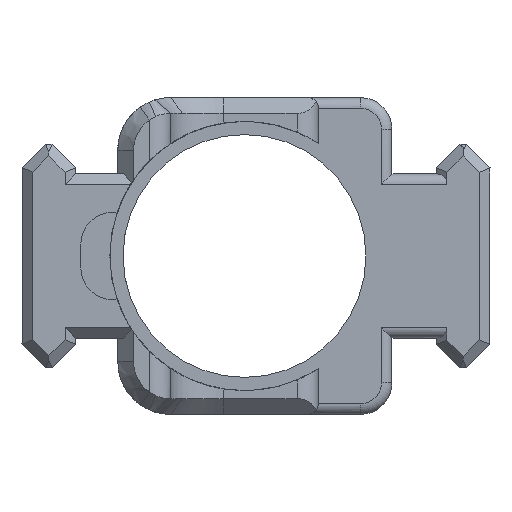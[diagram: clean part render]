
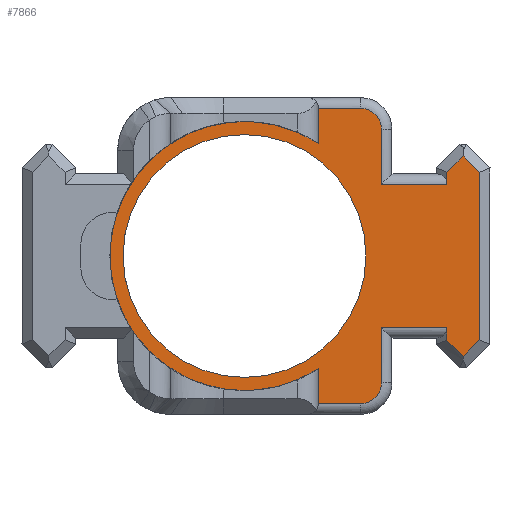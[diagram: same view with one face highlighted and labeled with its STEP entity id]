
A CAD part, left-side view. The second image highlights one B-rep face of the part: STEP entity #7866.
In plain terms, the highlighted planar face has unit normal (-1, 0, 0).
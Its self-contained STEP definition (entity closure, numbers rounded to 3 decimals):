
#35=FACE_BOUND('',#786,.T.);
#176=CIRCLE('',#8368,12.75);
#184=CIRCLE('',#8390,2.);
#185=CIRCLE('',#8391,2.);
#186=CIRCLE('',#8392,11.5);
#327=FACE_OUTER_BOUND('',#785,.T.);
#785=EDGE_LOOP('',(#5769,#5770,#5771,#5772,#5773,#5774,#5775,#5776,#5777,
#5778,#5779,#5780,#5781,#5782,#5783,#5784,#5785,#5786));
#786=EDGE_LOOP('',(#5787));
#1500=LINE('',#12039,#2532);
#1501=LINE('',#12043,#2533);
#1504=LINE('',#12059,#2536);
#1508=LINE('',#12072,#2540);
#1509=LINE('',#12074,#2541);
#1510=LINE('',#12076,#2542);
#1511=LINE('',#12078,#2543);
#1512=LINE('',#12080,#2544);
#1513=LINE('',#12082,#2545);
#1514=LINE('',#12084,#2546);
#1515=LINE('',#12086,#2547);
#1516=LINE('',#12088,#2548);
#1517=LINE('',#12090,#2549);
#1518=LINE('',#12092,#2550);
#1519=LINE('',#12095,#2551);
#2532=VECTOR('',#9451,10.);
#2533=VECTOR('',#9456,10.);
#2536=VECTOR('',#9467,10.);
#2540=VECTOR('',#9481,10.);
#2541=VECTOR('',#9482,10.);
#2542=VECTOR('',#9483,10.);
#2543=VECTOR('',#9484,10.);
#2544=VECTOR('',#9485,10.);
#2545=VECTOR('',#9486,10.);
#2546=VECTOR('',#9487,10.);
#2547=VECTOR('',#9488,10.);
#2548=VECTOR('',#9489,10.);
#2549=VECTOR('',#9490,10.);
#2550=VECTOR('',#9491,10.);
#2551=VECTOR('',#9494,10.);
#3503=VERTEX_POINT('',#11846);
#3510=VERTEX_POINT('',#11880);
#3511=VERTEX_POINT('',#11882);
#3533=VERTEX_POINT('',#12041);
#3536=VERTEX_POINT('',#12053);
#3539=VERTEX_POINT('',#12069);
#3540=VERTEX_POINT('',#12071);
#3541=VERTEX_POINT('',#12073);
#3542=VERTEX_POINT('',#12075);
#3543=VERTEX_POINT('',#12077);
#3544=VERTEX_POINT('',#12079);
#3545=VERTEX_POINT('',#12081);
#3546=VERTEX_POINT('',#12083);
#3547=VERTEX_POINT('',#12085);
#3548=VERTEX_POINT('',#12087);
#3549=VERTEX_POINT('',#12089);
#3550=VERTEX_POINT('',#12091);
#3551=VERTEX_POINT('',#12093);
#3552=VERTEX_POINT('',#12096);
#4323=EDGE_CURVE('',#3510,#3511,#176,.T.);
#4346=EDGE_CURVE('',#3510,#3503,#1500,.T.);
#4348=EDGE_CURVE('',#3533,#3503,#1501,.T.);
#4354=EDGE_CURVE('',#3536,#3511,#1504,.T.);
#4359=EDGE_CURVE('',#3539,#3533,#184,.T.);
#4360=EDGE_CURVE('',#3540,#3539,#1508,.T.);
#4361=EDGE_CURVE('',#3541,#3540,#1509,.T.);
#4362=EDGE_CURVE('',#3542,#3541,#1510,.T.);
#4363=EDGE_CURVE('',#3543,#3542,#1511,.T.);
#4364=EDGE_CURVE('',#3544,#3543,#1512,.T.);
#4365=EDGE_CURVE('',#3545,#3544,#1513,.T.);
#4366=EDGE_CURVE('',#3546,#3545,#1514,.T.);
#4367=EDGE_CURVE('',#3547,#3546,#1515,.T.);
#4368=EDGE_CURVE('',#3548,#3547,#1516,.T.);
#4369=EDGE_CURVE('',#3549,#3548,#1517,.T.);
#4370=EDGE_CURVE('',#3550,#3549,#1518,.T.);
#4371=EDGE_CURVE('',#3551,#3550,#185,.T.);
#4372=EDGE_CURVE('',#3536,#3551,#1519,.T.);
#4373=EDGE_CURVE('',#3552,#3552,#186,.F.);
#5769=ORIENTED_EDGE('',*,*,#4323,.F.);
#5770=ORIENTED_EDGE('',*,*,#4346,.T.);
#5771=ORIENTED_EDGE('',*,*,#4348,.F.);
#5772=ORIENTED_EDGE('',*,*,#4359,.F.);
#5773=ORIENTED_EDGE('',*,*,#4360,.F.);
#5774=ORIENTED_EDGE('',*,*,#4361,.F.);
#5775=ORIENTED_EDGE('',*,*,#4362,.F.);
#5776=ORIENTED_EDGE('',*,*,#4363,.F.);
#5777=ORIENTED_EDGE('',*,*,#4364,.F.);
#5778=ORIENTED_EDGE('',*,*,#4365,.F.);
#5779=ORIENTED_EDGE('',*,*,#4366,.F.);
#5780=ORIENTED_EDGE('',*,*,#4367,.F.);
#5781=ORIENTED_EDGE('',*,*,#4368,.F.);
#5782=ORIENTED_EDGE('',*,*,#4369,.F.);
#5783=ORIENTED_EDGE('',*,*,#4370,.F.);
#5784=ORIENTED_EDGE('',*,*,#4371,.F.);
#5785=ORIENTED_EDGE('',*,*,#4372,.F.);
#5786=ORIENTED_EDGE('',*,*,#4354,.T.);
#5787=ORIENTED_EDGE('',*,*,#4373,.T.);
#7442=PLANE('',#8389);
#7866=ADVANCED_FACE('',(#327,#35),#7442,.T.);
#8368=AXIS2_PLACEMENT_3D('',#11883,#9422,#9423);
#8389=AXIS2_PLACEMENT_3D('',#12068,#9477,#9478);
#8390=AXIS2_PLACEMENT_3D('',#12070,#9479,#9480);
#8391=AXIS2_PLACEMENT_3D('',#12094,#9492,#9493);
#8392=AXIS2_PLACEMENT_3D('',#12097,#9495,#9496);
#9422=DIRECTION('center_axis',(1.,0.,0.));
#9423=DIRECTION('ref_axis',(0.,-1.,0.));
#9451=DIRECTION('',(0.,0.,-1.));
#9456=DIRECTION('',(0.,1.,0.));
#9467=DIRECTION('',(0.,0.,-1.));
#9477=DIRECTION('center_axis',(-1.,0.,0.));
#9478=DIRECTION('ref_axis',(0.,-1.,0.));
#9479=DIRECTION('center_axis',(1.,0.,0.));
#9480=DIRECTION('ref_axis',(0.,-0.707,-0.707));
#9481=DIRECTION('',(0.,0.,-1.));
#9482=DIRECTION('',(0.,1.,0.));
#9483=DIRECTION('',(0.,0.,1.));
#9484=DIRECTION('',(0.,0.707,0.707));
#9485=DIRECTION('',(0.,0.707,-0.707));
#9486=DIRECTION('',(0.,0.,-1.));
#9487=DIRECTION('',(0.,-0.707,-0.707));
#9488=DIRECTION('',(0.,-0.707,0.707));
#9489=DIRECTION('',(0.,0.,1.));
#9490=DIRECTION('',(0.,-1.,0.));
#9491=DIRECTION('',(0.,0.,-1.));
#9492=DIRECTION('center_axis',(1.,0.,0.));
#9493=DIRECTION('ref_axis',(0.,-0.707,0.707));
#9494=DIRECTION('',(0.,-1.,0.));
#9495=DIRECTION('center_axis',(-1.,0.,0.));
#9496=DIRECTION('ref_axis',(0.,1.,0.));
#11846=CARTESIAN_POINT('',(-1.,-123.985,1.));
#11880=CARTESIAN_POINT('',(-1.,-123.985,4.334));
#11882=CARTESIAN_POINT('',(-1.,-123.985,25.666));
#11883=CARTESIAN_POINT('Origin',(-1.,-117.,15.));
#12039=CARTESIAN_POINT('',(-1.,-123.985,0.));
#12041=CARTESIAN_POINT('',(-1.,-127.97,1.));
#12043=CARTESIAN_POINT('',(-1.,-108.5,1.));
#12053=CARTESIAN_POINT('',(-1.,-123.985,29.));
#12059=CARTESIAN_POINT('',(-1.,-123.985,12.682));
#12068=CARTESIAN_POINT('Origin',(-1.,-100.,0.));
#12069=CARTESIAN_POINT('',(-1.,-129.97,3.));
#12070=CARTESIAN_POINT('Origin',(-1.,-127.97,3.));
#12071=CARTESIAN_POINT('',(-1.,-129.97,8.219));
#12072=CARTESIAN_POINT('',(-1.,-129.97,-0.187));
#12073=CARTESIAN_POINT('',(-1.,-136.173,8.219));
#12074=CARTESIAN_POINT('',(-1.,-117.586,8.219));
#12075=CARTESIAN_POINT('',(-1.,-136.173,7.001));
#12076=CARTESIAN_POINT('',(-1.,-136.173,3.324));
#12077=CARTESIAN_POINT('',(-1.,-137.713,5.521));
#12078=CARTESIAN_POINT('',(-1.,-128.748,14.486));
#12079=CARTESIAN_POINT('',(-1.,-139.253,7.061));
#12080=CARTESIAN_POINT('',(-1.,-126.703,-5.488));
#12081=CARTESIAN_POINT('',(-1.,-139.253,22.921));
#12082=CARTESIAN_POINT('',(-1.,-139.253,3.324));
#12083=CARTESIAN_POINT('',(-1.,-137.7,24.474));
#12084=CARTESIAN_POINT('',(-1.,-135.316,26.857));
#12085=CARTESIAN_POINT('',(-1.,-136.173,22.947));
#12086=CARTESIAN_POINT('',(-1.,-122.358,9.132));
#12087=CARTESIAN_POINT('',(-1.,-136.173,21.79));
#12088=CARTESIAN_POINT('',(-1.,-136.173,11.382));
#12089=CARTESIAN_POINT('',(-1.,-129.97,21.79));
#12090=CARTESIAN_POINT('',(-1.,-115.465,21.79));
#12091=CARTESIAN_POINT('',(-1.,-129.97,27.));
#12092=CARTESIAN_POINT('',(-1.,-129.97,-0.187));
#12093=CARTESIAN_POINT('',(-1.,-127.97,29.));
#12094=CARTESIAN_POINT('Origin',(-1.,-127.97,27.));
#12095=CARTESIAN_POINT('',(-1.,-108.5,29.));
#12096=CARTESIAN_POINT('',(-1.,-128.5,15.));
#12097=CARTESIAN_POINT('Origin',(-1.,-117.,15.));
